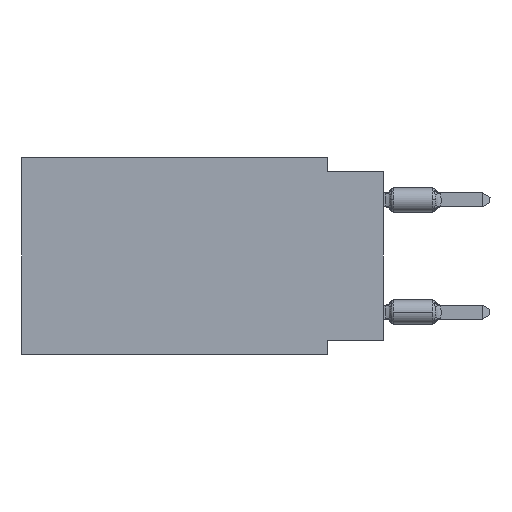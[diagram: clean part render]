
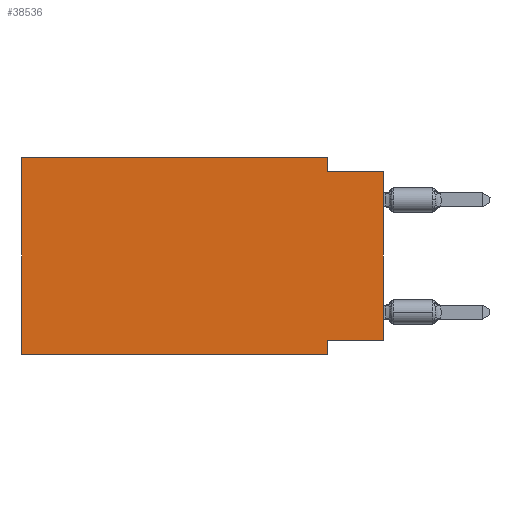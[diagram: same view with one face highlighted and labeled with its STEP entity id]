
A CAD part, left-side view. The second image highlights one B-rep face of the part: STEP entity #38536.
In plain terms, the highlighted planar face has unit normal (-1, 0, 0).
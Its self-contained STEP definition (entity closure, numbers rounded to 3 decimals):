
#63 = ORIENTED_EDGE ( 'NONE', *, *, #3164, .F. ) ;
#975 = DIRECTION ( 'NONE',  ( 0., -1., 0. ) ) ;
#1119 = CARTESIAN_POINT ( 'NONE',  ( 0., 16.383, 0. ) ) ;
#1657 = EDGE_CURVE ( 'NONE', #19315, #48861, #32732, .T. ) ;
#3138 = VECTOR ( 'NONE', #5771, 1000. ) ;
#3164 = EDGE_CURVE ( 'NONE', #48861, #44733, #38205, .T. ) ;
#3495 = EDGE_CURVE ( 'NONE', #4263, #56481, #14847, .T. ) ;
#4263 = VERTEX_POINT ( 'NONE', #32129 ) ;
#5771 = DIRECTION ( 'NONE',  ( 0., 0., -1. ) ) ;
#5883 = DIRECTION ( 'NONE',  ( 0., 0., 1. ) ) ;
#7474 = DIRECTION ( 'NONE',  ( 0., -1., 0. ) ) ;
#7556 = VECTOR ( 'NONE', #15792, 1000. ) ;
#7672 = VERTEX_POINT ( 'NONE', #1119 ) ;
#8169 = EDGE_CURVE ( 'NONE', #56519, #4263, #50632, .T. ) ;
#9658 = LINE ( 'NONE', #26520, #29411 ) ;
#10538 = ORIENTED_EDGE ( 'NONE', *, *, #8169, .F. ) ;
#10733 = ORIENTED_EDGE ( 'NONE', *, *, #40438, .F. ) ;
#13879 = VECTOR ( 'NONE', #50783, 1000. ) ;
#14847 = LINE ( 'NONE', #41402, #26456 ) ;
#15792 = DIRECTION ( 'NONE',  ( 0., 0., -1. ) ) ;
#17270 = DIRECTION ( 'NONE',  ( 1., 0., 0. ) ) ;
#17341 = CARTESIAN_POINT ( 'NONE',  ( 0., 16.383, -8.89 ) ) ;
#19315 = VERTEX_POINT ( 'NONE', #57072 ) ;
#21902 = ORIENTED_EDGE ( 'NONE', *, *, #3495, .F. ) ;
#23568 = DIRECTION ( 'NONE',  ( 0., 1., 0. ) ) ;
#24186 = LINE ( 'NONE', #28910, #35652 ) ;
#24339 = CARTESIAN_POINT ( 'NONE',  ( 0., 16.383, -8.89 ) ) ;
#26088 = VERTEX_POINT ( 'NONE', #17341 ) ;
#26456 = VECTOR ( 'NONE', #975, 1000. ) ;
#26520 = CARTESIAN_POINT ( 'NONE',  ( 0., 16.383, 0. ) ) ;
#27234 = VECTOR ( 'NONE', #7474, 1000. ) ;
#27904 = ORIENTED_EDGE ( 'NONE', *, *, #29021, .T. ) ;
#28087 = CARTESIAN_POINT ( 'NONE',  ( 0., 16.383, 0. ) ) ;
#28515 = CARTESIAN_POINT ( 'NONE',  ( 0., 2.54, 0. ) ) ;
#28910 = CARTESIAN_POINT ( 'NONE',  ( 0., 0., 0. ) ) ;
#29021 = EDGE_CURVE ( 'NONE', #19315, #56481, #24186, .T. ) ;
#29371 = EDGE_CURVE ( 'NONE', #26088, #44733, #43484, .T. ) ;
#29411 = VECTOR ( 'NONE', #49793, 1000. ) ;
#31999 = DIRECTION ( 'NONE',  ( 0., 0., -1. ) ) ;
#32129 = CARTESIAN_POINT ( 'NONE',  ( 0., 2.54, -0.635 ) ) ;
#32732 = LINE ( 'NONE', #40992, #51616 ) ;
#34136 = CARTESIAN_POINT ( 'NONE',  ( 0., 0., -0.635 ) ) ;
#34505 = CARTESIAN_POINT ( 'NONE',  ( 0., 2.54, -8.255 ) ) ;
#35541 = CARTESIAN_POINT ( 'NONE',  ( 0., 16.383, 0. ) ) ;
#35652 = VECTOR ( 'NONE', #5883, 1000. ) ;
#37202 = LINE ( 'NONE', #28087, #13879 ) ;
#37956 = CARTESIAN_POINT ( 'NONE',  ( 0., 2.54, 0. ) ) ;
#38205 = LINE ( 'NONE', #56209, #7556 ) ;
#38536 = ADVANCED_FACE ( 'NONE', ( #53543 ), #40252, .F. ) ;
#40252 = PLANE ( 'NONE',  #57163 ) ;
#40438 = EDGE_CURVE ( 'NONE', #7672, #56519, #37202, .T. ) ;
#40992 = CARTESIAN_POINT ( 'NONE',  ( 0., 0., -8.255 ) ) ;
#41402 = CARTESIAN_POINT ( 'NONE',  ( 0., 0., -0.635 ) ) ;
#41678 = ORIENTED_EDGE ( 'NONE', *, *, #50461, .F. ) ;
#42437 = ORIENTED_EDGE ( 'NONE', *, *, #1657, .F. ) ;
#43484 = LINE ( 'NONE', #24339, #27234 ) ;
#44264 = EDGE_LOOP ( 'NONE', ( #27904, #21902, #10538, #10733, #41678, #57062, #63, #42437 ) ) ;
#44733 = VERTEX_POINT ( 'NONE', #51164 ) ;
#48861 = VERTEX_POINT ( 'NONE', #34505 ) ;
#49793 = DIRECTION ( 'NONE',  ( 0., 0., 1. ) ) ;
#50461 = EDGE_CURVE ( 'NONE', #26088, #7672, #9658, .T. ) ;
#50632 = LINE ( 'NONE', #28515, #3138 ) ;
#50783 = DIRECTION ( 'NONE',  ( 0., -1., 0. ) ) ;
#51164 = CARTESIAN_POINT ( 'NONE',  ( 0., 2.54, -8.89 ) ) ;
#51616 = VECTOR ( 'NONE', #23568, 1000. ) ;
#53543 = FACE_OUTER_BOUND ( 'NONE', #44264, .T. ) ;
#56209 = CARTESIAN_POINT ( 'NONE',  ( 0., 2.54, -8.89 ) ) ;
#56481 = VERTEX_POINT ( 'NONE', #34136 ) ;
#56519 = VERTEX_POINT ( 'NONE', #37956 ) ;
#57062 = ORIENTED_EDGE ( 'NONE', *, *, #29371, .T. ) ;
#57072 = CARTESIAN_POINT ( 'NONE',  ( 0., 0., -8.255 ) ) ;
#57163 = AXIS2_PLACEMENT_3D ( 'NONE', #35541, #17270, #31999 ) ;
